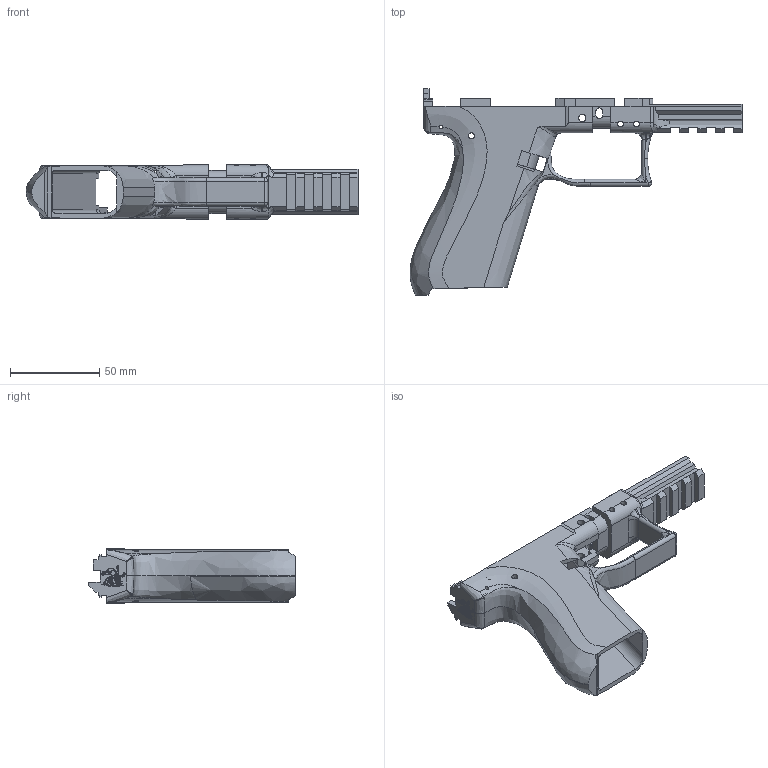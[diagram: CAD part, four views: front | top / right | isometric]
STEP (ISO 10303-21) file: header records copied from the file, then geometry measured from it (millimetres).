
FILE_DESCRIPTION (( 'STEP AP214' ), '1' );
FILE_NAME ('FrameBoi 1204.STEP', '2022-04-25T03:18:10', ( '' ), ( '' ), 'SwSTEP 2.0', 'SolidWorks 2019', '' );
FILE_SCHEMA (( 'AUTOMOTIVE_DESIGN' ));
Length unit declared in the file: millimetre
Products named in the file (1): FrameBoi 1204
Bounding box: 186.07 x 115.7 x 30.5 mm (x, y, z)
Volume: 84314.7 mm3; surface area: 47999.3 mm2
Topology: 1 solids, 1 shells, 3874 faces, 11516 edges, 7659 vertices
Faces by surface type: cylinder 3363, plane 453, bspline 48, torus 6, sphere 4
Entity records: 143674 total; most frequent: CARTESIAN_POINT 33657, DIRECTION 25641, ORIENTED_EDGE 23018, EDGE_CURVE 11509, AXIS2_PLACEMENT_3D 10539, VERTEX_POINT 7659, CIRCLE 6712, VECTOR 4563
